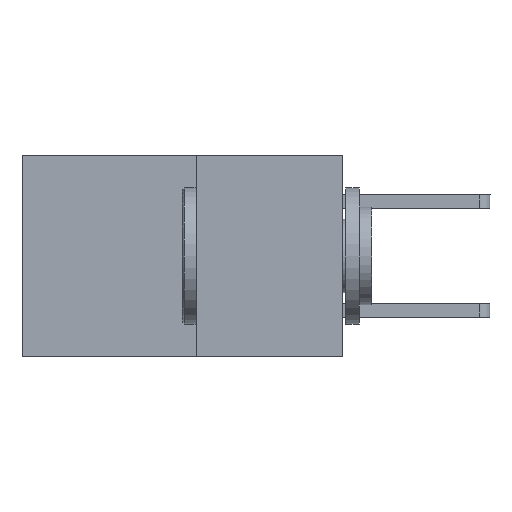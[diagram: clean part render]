
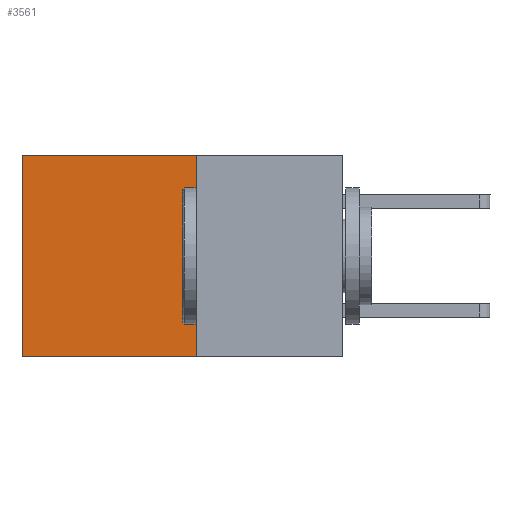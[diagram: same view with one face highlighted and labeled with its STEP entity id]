
A CAD part, left-side view. The second image highlights one B-rep face of the part: STEP entity #3561.
In plain terms, the highlighted planar face has unit normal (-1, 0, 0).
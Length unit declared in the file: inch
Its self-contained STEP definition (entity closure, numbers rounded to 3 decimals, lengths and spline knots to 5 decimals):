
#211 = AXIS2_PLACEMENT_3D ( 'NONE', #4298, #3646, #4339 ) ;
#417 = CARTESIAN_POINT ( 'NONE',  ( 0.277, 0.27, 0. ) ) ;
#466 = DIRECTION ( 'NONE',  ( 0., 1., 0. ) ) ;
#1103 = CARTESIAN_POINT ( 'NONE',  ( 0.277, 0.27, -0.37 ) ) ;
#1821 = LINE ( 'NONE', #8461, #4575 ) ;
#2052 = CARTESIAN_POINT ( 'NONE',  ( 0.277, 0.27, -0.37 ) ) ;
#2229 = VECTOR ( 'NONE', #466, 39.37008 ) ;
#2595 = CARTESIAN_POINT ( 'NONE',  ( 0.277, 0.27, -0.37 ) ) ;
#2661 = ORIENTED_EDGE ( 'NONE', *, *, #6545, .F. ) ;
#2753 = ORIENTED_EDGE ( 'NONE', *, *, #4088, .F. ) ;
#2817 = DIRECTION ( 'NONE',  ( 0., 0., -1. ) ) ;
#3240 = ORIENTED_EDGE ( 'NONE', *, *, #5078, .T. ) ;
#3277 = DIRECTION ( 'NONE',  ( 0., 0., -1. ) ) ;
#3381 = VERTEX_POINT ( 'NONE', #4503 ) ;
#3561 = ADVANCED_FACE ( 'NONE', ( #8267 ), #7621, .F. ) ;
#3586 = VECTOR ( 'NONE', #5216, 39.37008 ) ;
#3646 = DIRECTION ( 'NONE',  ( 1., 0., 0. ) ) ;
#3668 = VERTEX_POINT ( 'NONE', #1103 ) ;
#4088 = EDGE_CURVE ( 'NONE', #3381, #3668, #7917, .T. ) ;
#4298 = CARTESIAN_POINT ( 'NONE',  ( 0.277, 0.27, -0.37 ) ) ;
#4338 = VERTEX_POINT ( 'NONE', #4695 ) ;
#4339 = DIRECTION ( 'NONE',  ( 0., 0., -1. ) ) ;
#4503 = CARTESIAN_POINT ( 'NONE',  ( 0.277, 0.27, 0. ) ) ;
#4575 = VECTOR ( 'NONE', #3277, 39.37008 ) ;
#4695 = CARTESIAN_POINT ( 'NONE',  ( 0.277, 0.59, 0. ) ) ;
#5078 = EDGE_CURVE ( 'NONE', #3381, #4338, #7524, .T. ) ;
#5216 = DIRECTION ( 'NONE',  ( 0., 1., 0. ) ) ;
#5650 = EDGE_CURVE ( 'NONE', #4338, #6376, #1821, .T. ) ;
#5864 = LINE ( 'NONE', #2595, #3586 ) ;
#6376 = VERTEX_POINT ( 'NONE', #8241 ) ;
#6539 = VECTOR ( 'NONE', #2817, 39.37008 ) ;
#6545 = EDGE_CURVE ( 'NONE', #3668, #6376, #5864, .T. ) ;
#7524 = LINE ( 'NONE', #417, #2229 ) ;
#7621 = PLANE ( 'NONE',  #211 ) ;
#7831 = ORIENTED_EDGE ( 'NONE', *, *, #5650, .T. ) ;
#7917 = LINE ( 'NONE', #2052, #6539 ) ;
#8100 = EDGE_LOOP ( 'NONE', ( #7831, #2661, #2753, #3240 ) ) ;
#8241 = CARTESIAN_POINT ( 'NONE',  ( 0.277, 0.59, -0.37 ) ) ;
#8267 = FACE_OUTER_BOUND ( 'NONE', #8100, .T. ) ;
#8461 = CARTESIAN_POINT ( 'NONE',  ( 0.277, 0.59, -0.37 ) ) ;
